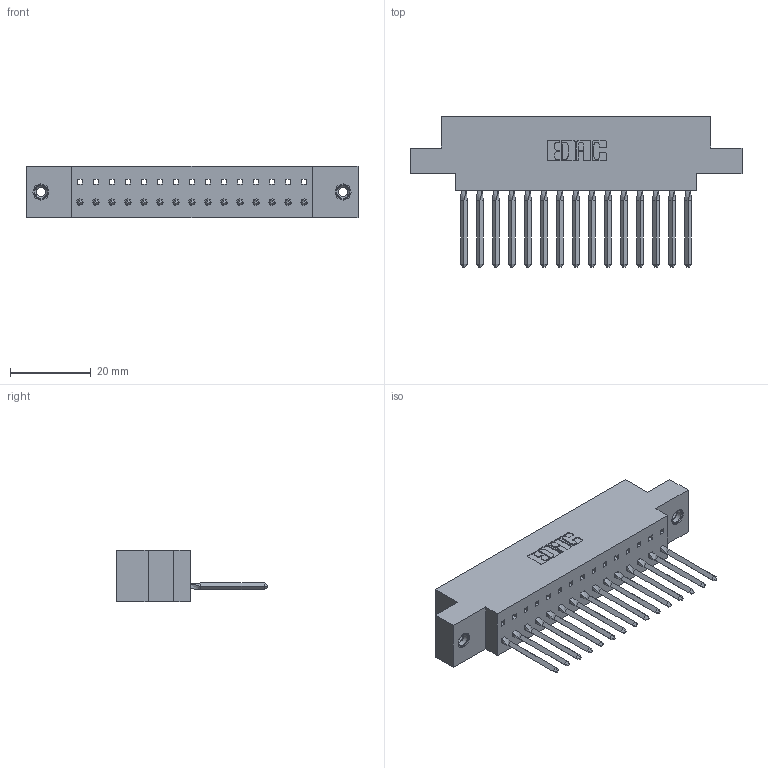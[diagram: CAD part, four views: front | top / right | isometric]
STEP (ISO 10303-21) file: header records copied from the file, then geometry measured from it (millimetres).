
FILE_DESCRIPTION (( 'STEP AP203' ), '1' );
FILE_NAME ('317-015-542-608.STEP', '2020-02-27T15:00:28', ( '' ), ( '' ), 'SwSTEP 2.0', 'SolidWorks 2016', '' );
FILE_SCHEMA (( 'CONFIG_CONTROL_DESIGN' ));
Length unit declared in the file: inch
Products named in the file (4): 317-290-003_542; 345-250-001_345-250-003-102; 317-015-542-608; 317 Part_.156 Dia - TI
Assembly tree (18 placements, depth 2):
  317-015-542-608
    317 Part_.156 Dia - TI
    317-290-003_542  x15
    345-250-001_345-250-003-102  x2
Bounding box: 82.14 x 37.34 x 12.7 mm (x, y, z)
Volume: 11964.5 mm3; surface area: 14013.5 mm2
Topology: 18 solids, 18 shells, 1287 faces, 3666 edges, 2366 vertices
Faces by surface type: plane 1050, cylinder 161, bspline 60, cone 12, torus 4
Entity records: 25172 total; most frequent: CARTESIAN_POINT 4677, ORIENTED_EDGE 4348, DIRECTION 3714, EDGE_CURVE 2174, LINE 1984, VECTOR 1984, VERTEX_POINT 1440, AXIS2_PLACEMENT_3D 865
